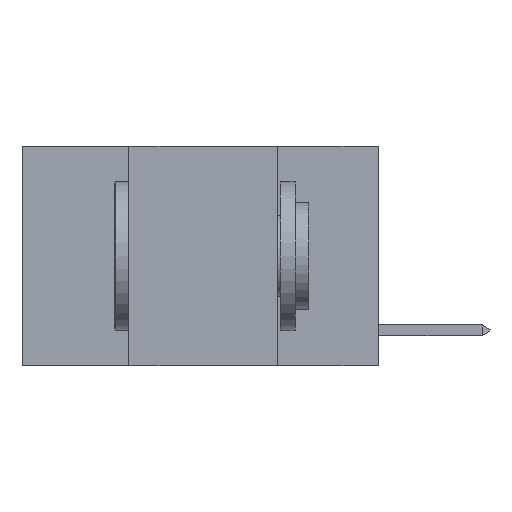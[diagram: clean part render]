
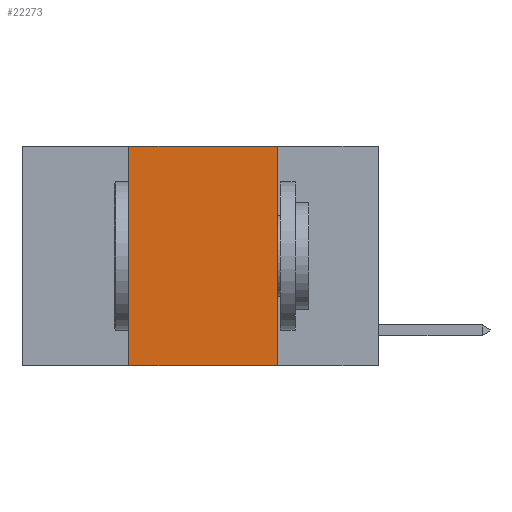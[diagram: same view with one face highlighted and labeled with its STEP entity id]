
A CAD part, left-side view. The second image highlights one B-rep face of the part: STEP entity #22273.
In plain terms, the highlighted planar face has unit normal (-1, 0, 0).
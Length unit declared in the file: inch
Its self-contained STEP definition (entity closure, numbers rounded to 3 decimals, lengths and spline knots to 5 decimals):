
#1646 = LINE ( 'NONE', #10858, #18853 ) ;
#1672 = DIRECTION ( 'NONE',  ( 0., 0., -1. ) ) ;
#1691 = EDGE_LOOP ( 'NONE', ( #7374, #20487, #11074, #8759 ) ) ;
#3537 = CARTESIAN_POINT ( 'NONE',  ( 0., 0.6, 0. ) ) ;
#3651 = AXIS2_PLACEMENT_3D ( 'NONE', #3537, #17863, #1672 ) ;
#3787 = EDGE_CURVE ( 'NONE', #17406, #22932, #3815, .T. ) ;
#3815 = LINE ( 'NONE', #21039, #6655 ) ;
#4035 = LINE ( 'NONE', #11143, #20988 ) ;
#4825 = VERTEX_POINT ( 'NONE', #18414 ) ;
#5145 = VECTOR ( 'NONE', #14556, 39.37008 ) ;
#5407 = FACE_OUTER_BOUND ( 'NONE', #1691, .T. ) ;
#5623 = DIRECTION ( 'NONE',  ( 0., -1., 0. ) ) ;
#5706 = CARTESIAN_POINT ( 'NONE',  ( 0., 0.6, -0.37 ) ) ;
#6655 = VECTOR ( 'NONE', #12534, 39.37008 ) ;
#7374 = ORIENTED_EDGE ( 'NONE', *, *, #17391, .F. ) ;
#8499 = EDGE_CURVE ( 'NONE', #22932, #4825, #1646, .T. ) ;
#8759 = ORIENTED_EDGE ( 'NONE', *, *, #9028, .T. ) ;
#9028 = EDGE_CURVE ( 'NONE', #17406, #20402, #11531, .T. ) ;
#9387 = CARTESIAN_POINT ( 'NONE',  ( 0., 0.42, -0.37 ) ) ;
#10858 = CARTESIAN_POINT ( 'NONE',  ( 0., 0.6, 0. ) ) ;
#11074 = ORIENTED_EDGE ( 'NONE', *, *, #3787, .F. ) ;
#11143 = CARTESIAN_POINT ( 'NONE',  ( 0., 0.17, 0. ) ) ;
#11531 = LINE ( 'NONE', #5706, #5145 ) ;
#11660 = CARTESIAN_POINT ( 'NONE',  ( 0., 0.17, -0.37 ) ) ;
#12534 = DIRECTION ( 'NONE',  ( 0., 0., 1. ) ) ;
#14556 = DIRECTION ( 'NONE',  ( 0., -1., 0. ) ) ;
#15580 = CARTESIAN_POINT ( 'NONE',  ( 0., 0.42, 0. ) ) ;
#17391 = EDGE_CURVE ( 'NONE', #4825, #20402, #4035, .T. ) ;
#17406 = VERTEX_POINT ( 'NONE', #9387 ) ;
#17863 = DIRECTION ( 'NONE',  ( 1., 0., 0. ) ) ;
#18247 = DIRECTION ( 'NONE',  ( 0., 0., -1. ) ) ;
#18414 = CARTESIAN_POINT ( 'NONE',  ( 0., 0.17, 0. ) ) ;
#18853 = VECTOR ( 'NONE', #5623, 39.37008 ) ;
#19614 = PLANE ( 'NONE',  #3651 ) ;
#20402 = VERTEX_POINT ( 'NONE', #11660 ) ;
#20487 = ORIENTED_EDGE ( 'NONE', *, *, #8499, .F. ) ;
#20988 = VECTOR ( 'NONE', #18247, 39.37008 ) ;
#21039 = CARTESIAN_POINT ( 'NONE',  ( 0., 0.42, 0. ) ) ;
#22273 = ADVANCED_FACE ( 'NONE', ( #5407 ), #19614, .F. ) ;
#22932 = VERTEX_POINT ( 'NONE', #15580 ) ;
